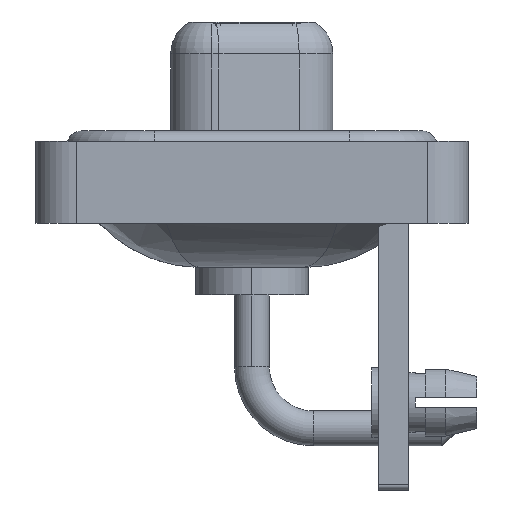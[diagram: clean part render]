
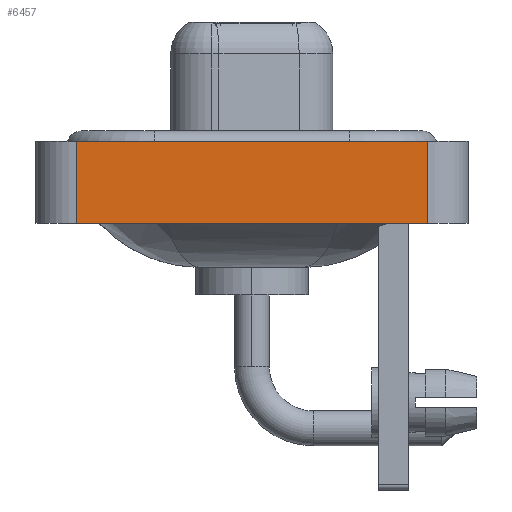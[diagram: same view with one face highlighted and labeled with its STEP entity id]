
A CAD part, left-side view. The second image highlights one B-rep face of the part: STEP entity #6457.
In plain terms, the highlighted planar face has unit normal (-1, 0, 0).
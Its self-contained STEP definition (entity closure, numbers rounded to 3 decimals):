
#408 = CARTESIAN_POINT ( 'NONE',  ( -7.25, -8.55, 0.4 ) ) ;
#873 = AXIS2_PLACEMENT_3D ( 'NONE', #12718, #11138, #18918 ) ;
#925 = LINE ( 'NONE', #18902, #4772 ) ;
#2385 = VECTOR ( 'NONE', #13412, 1000. ) ;
#2669 = ORIENTED_EDGE ( 'NONE', *, *, #13558, .F. ) ;
#2714 = CARTESIAN_POINT ( 'NONE',  ( -7.25, 8.55, 0.4 ) ) ;
#3719 = VERTEX_POINT ( 'NONE', #10627 ) ;
#4423 = EDGE_CURVE ( 'NONE', #18686, #3719, #6767, .T. ) ;
#4772 = VECTOR ( 'NONE', #11426, 1000. ) ;
#4909 = CARTESIAN_POINT ( 'NONE',  ( -7.25, 8.55, -3.6 ) ) ;
#6457 = ADVANCED_FACE ( 'NONE', ( #11044 ), #15565, .T. ) ;
#6767 = LINE ( 'NONE', #14032, #9329 ) ;
#7536 = CARTESIAN_POINT ( 'NONE',  ( -7.25, -8.55, -3.6 ) ) ;
#8162 = LINE ( 'NONE', #408, #8836 ) ;
#8251 = DIRECTION ( 'NONE',  ( 0., 0., 1. ) ) ;
#8836 = VECTOR ( 'NONE', #18381, 1000. ) ;
#8984 = VERTEX_POINT ( 'NONE', #2714 ) ;
#9329 = VECTOR ( 'NONE', #8251, 1000. ) ;
#10438 = EDGE_CURVE ( 'NONE', #11509, #18686, #14893, .T. ) ;
#10627 = CARTESIAN_POINT ( 'NONE',  ( -7.25, -8.55, 0.4 ) ) ;
#10731 = ORIENTED_EDGE ( 'NONE', *, *, #10438, .T. ) ;
#11044 = FACE_OUTER_BOUND ( 'NONE', #14037, .T. ) ;
#11138 = DIRECTION ( 'NONE',  ( -1., 0., 0. ) ) ;
#11158 = ORIENTED_EDGE ( 'NONE', *, *, #4423, .T. ) ;
#11426 = DIRECTION ( 'NONE',  ( 0., 0., 1. ) ) ;
#11509 = VERTEX_POINT ( 'NONE', #4909 ) ;
#12718 = CARTESIAN_POINT ( 'NONE',  ( -7.25, -8.55, -3.6 ) ) ;
#12910 = CARTESIAN_POINT ( 'NONE',  ( -7.25, -8.55, -3.6 ) ) ;
#13412 = DIRECTION ( 'NONE',  ( 0., -1., 0. ) ) ;
#13558 = EDGE_CURVE ( 'NONE', #11509, #8984, #925, .T. ) ;
#14032 = CARTESIAN_POINT ( 'NONE',  ( -7.25, -8.55, -3.6 ) ) ;
#14037 = EDGE_LOOP ( 'NONE', ( #11158, #15446, #2669, #10731 ) ) ;
#14893 = LINE ( 'NONE', #7536, #2385 ) ;
#15446 = ORIENTED_EDGE ( 'NONE', *, *, #16794, .F. ) ;
#15565 = PLANE ( 'NONE',  #873 ) ;
#16794 = EDGE_CURVE ( 'NONE', #8984, #3719, #8162, .T. ) ;
#18381 = DIRECTION ( 'NONE',  ( 0., -1., 0. ) ) ;
#18686 = VERTEX_POINT ( 'NONE', #12910 ) ;
#18902 = CARTESIAN_POINT ( 'NONE',  ( -7.25, 8.55, -3.6 ) ) ;
#18918 = DIRECTION ( 'NONE',  ( 0., 0., 1. ) ) ;
